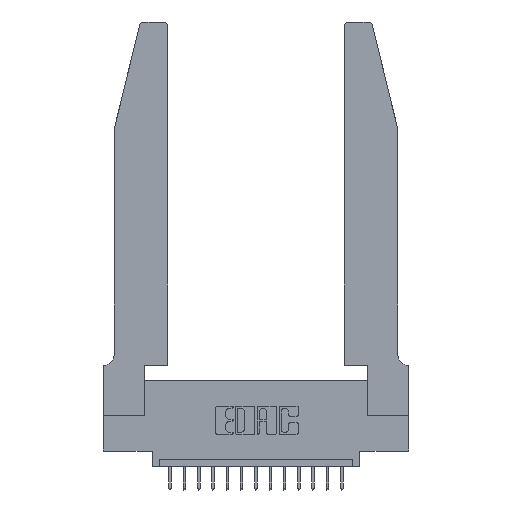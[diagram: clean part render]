
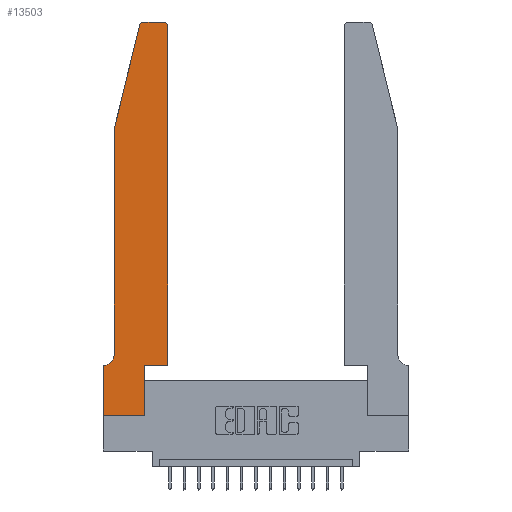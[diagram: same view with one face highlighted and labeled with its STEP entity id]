
A CAD part, top view. The second image highlights one B-rep face of the part: STEP entity #13503.
In plain terms, the highlighted planar face has unit normal (0, 0, 1).
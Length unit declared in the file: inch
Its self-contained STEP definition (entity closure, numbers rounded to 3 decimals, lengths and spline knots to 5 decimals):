
#20 = LINE ( 'NONE', #2428, #7411 ) ;
#112 = CARTESIAN_POINT ( 'NONE',  ( 0.284, 2.75, 0.37 ) ) ;
#328 = CARTESIAN_POINT ( 'NONE',  ( 0.2865, 0., 0.37 ) ) ;
#540 = CARTESIAN_POINT ( 'NONE',  ( 0.4505, 0.35, 0.37 ) ) ;
#969 = CARTESIAN_POINT ( 'NONE',  ( 0.0755, 0.35, 0.37 ) ) ;
#1018 = LINE ( 'NONE', #540, #13800 ) ;
#1434 = CARTESIAN_POINT ( 'NONE',  ( 0.0055, 0.35, 0.37 ) ) ;
#1737 = VERTEX_POINT ( 'NONE', #112 ) ;
#1787 = CIRCLE ( 'NONE', #3747, 0.03 ) ;
#1940 = VECTOR ( 'NONE', #14489, 39.37008 ) ;
#2129 = DIRECTION ( 'NONE',  ( 0., 1., 0. ) ) ;
#2345 = VERTEX_POINT ( 'NONE', #3545 ) ;
#2428 = CARTESIAN_POINT ( 'NONE',  ( 0.0755, 2., 0.37 ) ) ;
#2628 = DIRECTION ( 'NONE',  ( 1., 0., 0. ) ) ;
#2784 = DIRECTION ( 'NONE',  ( 0., 0., 1. ) ) ;
#2836 = EDGE_CURVE ( 'NONE', #17945, #4986, #12989, .T. ) ;
#2914 = VERTEX_POINT ( 'NONE', #7362 ) ;
#2955 = LINE ( 'NONE', #4536, #7845 ) ;
#3472 = ORIENTED_EDGE ( 'NONE', *, *, #5403, .T. ) ;
#3545 = CARTESIAN_POINT ( 'NONE',  ( 0.4205, 2.75, 0.37 ) ) ;
#3747 = AXIS2_PLACEMENT_3D ( 'NONE', #8851, #7222, #2628 ) ;
#3862 = DIRECTION ( 'NONE',  ( 0., 0., 1. ) ) ;
#4127 = VECTOR ( 'NONE', #2129, 39.37008 ) ;
#4255 = DIRECTION ( 'NONE',  ( -0.239, -0.971, 0. ) ) ;
#4270 = CIRCLE ( 'NONE', #6868, 0.03 ) ;
#4364 = DIRECTION ( 'NONE',  ( -1., 0., 0. ) ) ;
#4437 = ORIENTED_EDGE ( 'NONE', *, *, #11675, .T. ) ;
#4440 = AXIS2_PLACEMENT_3D ( 'NONE', #5781, #2784, #8505 ) ;
#4468 = CARTESIAN_POINT ( 'NONE',  ( 0., 0., 0.37 ) ) ;
#4536 = CARTESIAN_POINT ( 'NONE',  ( 0.2605, 2.75, 0.37 ) ) ;
#4650 = LINE ( 'NONE', #969, #8209 ) ;
#4740 = VECTOR ( 'NONE', #11569, 39.37008 ) ;
#4741 = EDGE_CURVE ( 'NONE', #16631, #9617, #4650, .T. ) ;
#4986 = VERTEX_POINT ( 'NONE', #328 ) ;
#5329 = DIRECTION ( 'NONE',  ( 0., -1., 0. ) ) ;
#5403 = EDGE_CURVE ( 'NONE', #16613, #7409, #1018, .T. ) ;
#5429 = CARTESIAN_POINT ( 'NONE',  ( 0.2865, 0.35, 0.37 ) ) ;
#5781 = CARTESIAN_POINT ( 'NONE',  ( 0., 0.35, 0.37 ) ) ;
#5917 = ORIENTED_EDGE ( 'NONE', *, *, #7266, .T. ) ;
#5946 = CARTESIAN_POINT ( 'NONE',  ( 0., 0., 0.37 ) ) ;
#6252 = ORIENTED_EDGE ( 'NONE', *, *, #14519, .T. ) ;
#6642 = VERTEX_POINT ( 'NONE', #5429 ) ;
#6653 = LINE ( 'NONE', #4468, #1940 ) ;
#6661 = CARTESIAN_POINT ( 'NONE',  ( 0.4505, 2.72, 0.37 ) ) ;
#6868 = AXIS2_PLACEMENT_3D ( 'NONE', #18259, #3862, #8154 ) ;
#6869 = DIRECTION ( 'NONE',  ( 0., 1., 0. ) ) ;
#7046 = CARTESIAN_POINT ( 'NONE',  ( 0.0055, 0.42, 0.37 ) ) ;
#7222 = DIRECTION ( 'NONE',  ( 0., 0., 1. ) ) ;
#7266 = EDGE_CURVE ( 'NONE', #4986, #6642, #15119, .T. ) ;
#7362 = CARTESIAN_POINT ( 'NONE',  ( 0.0755, 0.42, 0.37 ) ) ;
#7409 = VERTEX_POINT ( 'NONE', #6661 ) ;
#7411 = VECTOR ( 'NONE', #5329, 39.37008 ) ;
#7845 = VECTOR ( 'NONE', #11882, 39.37008 ) ;
#7882 = ORIENTED_EDGE ( 'NONE', *, *, #17534, .T. ) ;
#7988 = EDGE_CURVE ( 'NONE', #10020, #2914, #20, .T. ) ;
#8154 = DIRECTION ( 'NONE',  ( 1., 0., 0. ) ) ;
#8209 = VECTOR ( 'NONE', #9524, 39.37008 ) ;
#8455 = DIRECTION ( 'NONE',  ( 0., 0., -1. ) ) ;
#8505 = DIRECTION ( 'NONE',  ( 1., 0., 0. ) ) ;
#8851 = CARTESIAN_POINT ( 'NONE',  ( 0.4205, 2.72, 0.37 ) ) ;
#9103 = EDGE_CURVE ( 'NONE', #7409, #2345, #1787, .T. ) ;
#9524 = DIRECTION ( 'NONE',  ( -1., 0., 0. ) ) ;
#9617 = VERTEX_POINT ( 'NONE', #11745 ) ;
#10020 = VERTEX_POINT ( 'NONE', #13754 ) ;
#10031 = CARTESIAN_POINT ( 'NONE',  ( 0.0755, 2., 0.37 ) ) ;
#10073 = ORIENTED_EDGE ( 'NONE', *, *, #4741, .T. ) ;
#10903 = EDGE_LOOP ( 'NONE', ( #13642, #7882, #4437, #14954, #6252, #10073, #17976, #14787, #5917, #10996, #3472, #17528 ) ) ;
#10906 = EDGE_CURVE ( 'NONE', #2345, #1737, #2955, .T. ) ;
#10996 = ORIENTED_EDGE ( 'NONE', *, *, #18223, .T. ) ;
#11460 = CARTESIAN_POINT ( 'NONE',  ( 0.4505, 0.35, 0.37 ) ) ;
#11515 = CARTESIAN_POINT ( 'NONE',  ( 0.4505, 0.35, 0.37 ) ) ;
#11569 = DIRECTION ( 'NONE',  ( 1., 0., 0. ) ) ;
#11675 = EDGE_CURVE ( 'NONE', #12748, #10020, #12778, .T. ) ;
#11745 = CARTESIAN_POINT ( 'NONE',  ( 0., 0.35, 0.37 ) ) ;
#11882 = DIRECTION ( 'NONE',  ( -1., 0., 0. ) ) ;
#12540 = CARTESIAN_POINT ( 'NONE',  ( 0.25487, 2.72718, 0.37 ) ) ;
#12748 = VERTEX_POINT ( 'NONE', #12540 ) ;
#12778 = LINE ( 'NONE', #10031, #18463 ) ;
#12989 = LINE ( 'NONE', #5946, #4740 ) ;
#13124 = FACE_OUTER_BOUND ( 'NONE', #10903, .T. ) ;
#13503 = ADVANCED_FACE ( 'NONE', ( #13124 ), #17358, .T. ) ;
#13520 = EDGE_CURVE ( 'NONE', #9617, #17945, #6653, .T. ) ;
#13542 = CARTESIAN_POINT ( 'NONE',  ( 0., 0., 0.37 ) ) ;
#13642 = ORIENTED_EDGE ( 'NONE', *, *, #10906, .T. ) ;
#13754 = CARTESIAN_POINT ( 'NONE',  ( 0.0755, 2., 0.37 ) ) ;
#13800 = VECTOR ( 'NONE', #6869, 39.37008 ) ;
#13877 = LINE ( 'NONE', #11515, #16835 ) ;
#14032 = CIRCLE ( 'NONE', #15518, 0.07 ) ;
#14489 = DIRECTION ( 'NONE',  ( 0., -1., 0. ) ) ;
#14519 = EDGE_CURVE ( 'NONE', #2914, #16631, #14032, .T. ) ;
#14787 = ORIENTED_EDGE ( 'NONE', *, *, #2836, .T. ) ;
#14954 = ORIENTED_EDGE ( 'NONE', *, *, #7988, .T. ) ;
#15119 = LINE ( 'NONE', #18024, #4127 ) ;
#15518 = AXIS2_PLACEMENT_3D ( 'NONE', #7046, #8455, #4364 ) ;
#15821 = DIRECTION ( 'NONE',  ( 1., 0., 0. ) ) ;
#16613 = VERTEX_POINT ( 'NONE', #11460 ) ;
#16631 = VERTEX_POINT ( 'NONE', #1434 ) ;
#16835 = VECTOR ( 'NONE', #15821, 39.37008 ) ;
#17358 = PLANE ( 'NONE',  #4440 ) ;
#17528 = ORIENTED_EDGE ( 'NONE', *, *, #9103, .T. ) ;
#17534 = EDGE_CURVE ( 'NONE', #1737, #12748, #4270, .T. ) ;
#17945 = VERTEX_POINT ( 'NONE', #13542 ) ;
#17976 = ORIENTED_EDGE ( 'NONE', *, *, #13520, .T. ) ;
#18024 = CARTESIAN_POINT ( 'NONE',  ( 0.2865, 0.35, 0.37 ) ) ;
#18223 = EDGE_CURVE ( 'NONE', #6642, #16613, #13877, .T. ) ;
#18259 = CARTESIAN_POINT ( 'NONE',  ( 0.284, 2.72, 0.37 ) ) ;
#18463 = VECTOR ( 'NONE', #4255, 39.37008 ) ;
